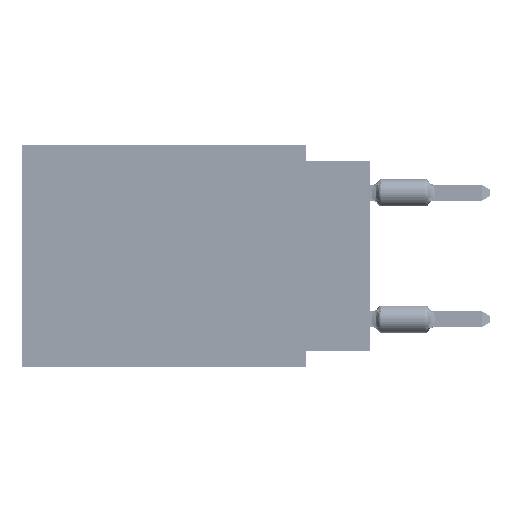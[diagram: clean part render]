
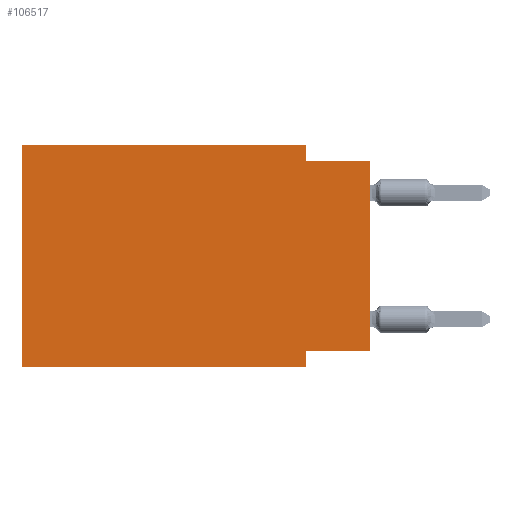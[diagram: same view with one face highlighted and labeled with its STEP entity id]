
A CAD part, left-side view. The second image highlights one B-rep face of the part: STEP entity #106517.
In plain terms, the highlighted planar face has unit normal (-1, 0, 0).
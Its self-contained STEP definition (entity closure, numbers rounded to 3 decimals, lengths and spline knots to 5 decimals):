
#2911 = AXIS2_PLACEMENT_3D ( 'NONE', #96667, #16622, #89060 ) ;
#6533 = CARTESIAN_POINT ( 'NONE',  ( 0., 0.1, -0.025 ) ) ;
#8916 = ORIENTED_EDGE ( 'NONE', *, *, #11316, .F. ) ;
#10604 = EDGE_CURVE ( 'NONE', #61680, #18512, #76156, .T. ) ;
#11316 = EDGE_CURVE ( 'NONE', #34468, #26269, #40670, .T. ) ;
#12662 = VECTOR ( 'NONE', #49862, 39.37008 ) ;
#13632 = ORIENTED_EDGE ( 'NONE', *, *, #10604, .T. ) ;
#16622 = DIRECTION ( 'NONE',  ( 1., 0., 0. ) ) ;
#18443 = CARTESIAN_POINT ( 'NONE',  ( 0., 0., -0.025 ) ) ;
#18512 = VERTEX_POINT ( 'NONE', #64182 ) ;
#21124 = VECTOR ( 'NONE', #103645, 39.37008 ) ;
#23330 = EDGE_LOOP ( 'NONE', ( #57793, #59727, #26467, #8916, #110135, #13632, #110671, #66618 ) ) ;
#23478 = VECTOR ( 'NONE', #88056, 39.37008 ) ;
#23601 = CARTESIAN_POINT ( 'NONE',  ( 0., 0.55, 0. ) ) ;
#24021 = VECTOR ( 'NONE', #111945, 39.37008 ) ;
#25741 = EDGE_CURVE ( 'NONE', #26269, #100056, #108854, .T. ) ;
#25765 = EDGE_CURVE ( 'NONE', #95819, #45155, #55109, .T. ) ;
#26269 = VERTEX_POINT ( 'NONE', #97553 ) ;
#26467 = ORIENTED_EDGE ( 'NONE', *, *, #25741, .F. ) ;
#30380 = CARTESIAN_POINT ( 'NONE',  ( 0., 0., -0.325 ) ) ;
#34468 = VERTEX_POINT ( 'NONE', #43704 ) ;
#35991 = DIRECTION ( 'NONE',  ( 0., -1., 0. ) ) ;
#40670 = LINE ( 'NONE', #93242, #24021 ) ;
#41102 = EDGE_CURVE ( 'NONE', #46942, #18512, #62499, .T. ) ;
#41664 = CARTESIAN_POINT ( 'NONE',  ( 0., 0.55, -0.35 ) ) ;
#42958 = FACE_OUTER_BOUND ( 'NONE', #23330, .T. ) ;
#43704 = CARTESIAN_POINT ( 'NONE',  ( 0., 0.55, 0. ) ) ;
#45155 = VERTEX_POINT ( 'NONE', #90231 ) ;
#45808 = DIRECTION ( 'NONE',  ( 0., 0., 1. ) ) ;
#46942 = VERTEX_POINT ( 'NONE', #92945 ) ;
#49862 = DIRECTION ( 'NONE',  ( 0., -1., 0. ) ) ;
#51840 = CARTESIAN_POINT ( 'NONE',  ( 0., 0., 0. ) ) ;
#54666 = LINE ( 'NONE', #18443, #80172 ) ;
#55109 = LINE ( 'NONE', #51840, #110991 ) ;
#57793 = ORIENTED_EDGE ( 'NONE', *, *, #25765, .T. ) ;
#58102 = LINE ( 'NONE', #23601, #21124 ) ;
#58299 = CARTESIAN_POINT ( 'NONE',  ( 0., 0., -0.325 ) ) ;
#59449 = LINE ( 'NONE', #58299, #105845 ) ;
#59727 = ORIENTED_EDGE ( 'NONE', *, *, #74979, .F. ) ;
#61029 = PLANE ( 'NONE',  #2911 ) ;
#61680 = VERTEX_POINT ( 'NONE', #101229 ) ;
#62499 = LINE ( 'NONE', #80062, #86058 ) ;
#64182 = CARTESIAN_POINT ( 'NONE',  ( 0., 0.1, -0.35 ) ) ;
#66618 = ORIENTED_EDGE ( 'NONE', *, *, #70768, .F. ) ;
#70768 = EDGE_CURVE ( 'NONE', #95819, #46942, #59449, .T. ) ;
#74979 = EDGE_CURVE ( 'NONE', #100056, #45155, #54666, .T. ) ;
#76156 = LINE ( 'NONE', #41664, #12662 ) ;
#80062 = CARTESIAN_POINT ( 'NONE',  ( 0., 0.1, -0.35 ) ) ;
#80172 = VECTOR ( 'NONE', #35991, 39.37008 ) ;
#81946 = EDGE_CURVE ( 'NONE', #61680, #34468, #58102, .T. ) ;
#86058 = VECTOR ( 'NONE', #106333, 39.37008 ) ;
#88056 = DIRECTION ( 'NONE',  ( 0., 0., -1. ) ) ;
#89060 = DIRECTION ( 'NONE',  ( 0., 0., -1. ) ) ;
#90231 = CARTESIAN_POINT ( 'NONE',  ( 0., 0., -0.025 ) ) ;
#92945 = CARTESIAN_POINT ( 'NONE',  ( 0., 0.1, -0.325 ) ) ;
#93242 = CARTESIAN_POINT ( 'NONE',  ( 0., 0.55, 0. ) ) ;
#95085 = DIRECTION ( 'NONE',  ( 0., 1., 0. ) ) ;
#95819 = VERTEX_POINT ( 'NONE', #30380 ) ;
#96667 = CARTESIAN_POINT ( 'NONE',  ( 0., 0.55, 0. ) ) ;
#97553 = CARTESIAN_POINT ( 'NONE',  ( 0., 0.1, 0. ) ) ;
#100056 = VERTEX_POINT ( 'NONE', #6533 ) ;
#101229 = CARTESIAN_POINT ( 'NONE',  ( 0., 0.55, -0.35 ) ) ;
#103645 = DIRECTION ( 'NONE',  ( 0., 0., 1. ) ) ;
#105845 = VECTOR ( 'NONE', #95085, 39.37008 ) ;
#106333 = DIRECTION ( 'NONE',  ( 0., 0., -1. ) ) ;
#106517 = ADVANCED_FACE ( 'NONE', ( #42958 ), #61029, .F. ) ;
#108284 = CARTESIAN_POINT ( 'NONE',  ( 0., 0.1, 0. ) ) ;
#108854 = LINE ( 'NONE', #108284, #23478 ) ;
#110135 = ORIENTED_EDGE ( 'NONE', *, *, #81946, .F. ) ;
#110671 = ORIENTED_EDGE ( 'NONE', *, *, #41102, .F. ) ;
#110991 = VECTOR ( 'NONE', #45808, 39.37008 ) ;
#111945 = DIRECTION ( 'NONE',  ( 0., -1., 0. ) ) ;
